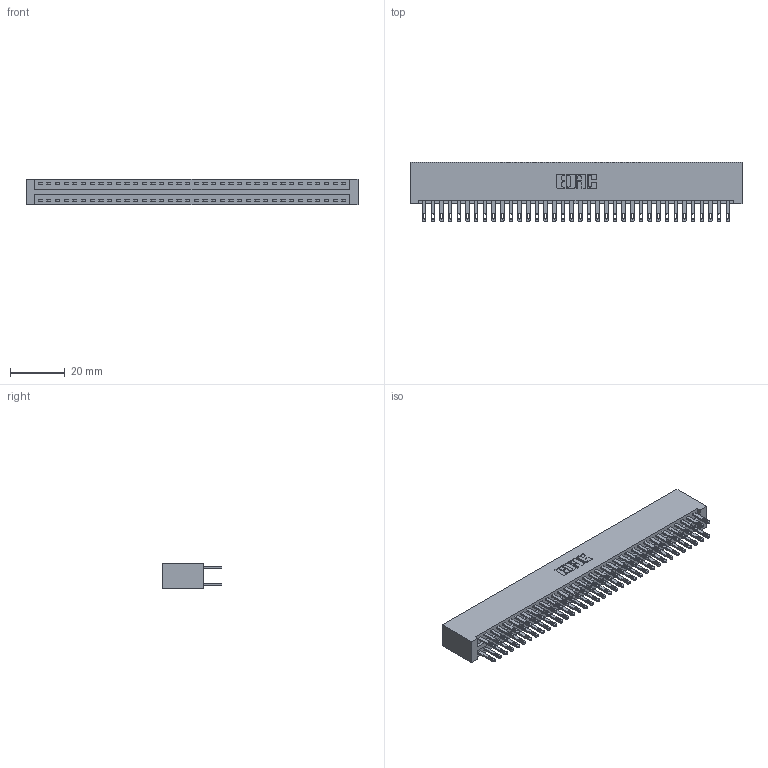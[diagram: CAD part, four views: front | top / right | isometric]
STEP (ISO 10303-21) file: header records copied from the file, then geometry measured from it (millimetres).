
FILE_DESCRIPTION (( 'STEP AP203' ), '1' );
FILE_NAME ('896-072-500-201.STEP', '2021-07-28T01:19:20', ( '' ), ( '' ), 'SwSTEP 2.0', 'SolidWorks 2020', '' );
FILE_SCHEMA (( 'CONFIG_CONTROL_DESIGN' ));
Length unit declared in the file: inch
Products named in the file (3): 345-292-001_345-293-100; 846 Part_No Mounting Lugs; 896-072-500-201
Assembly tree (73 placements, depth 2):
  896-072-500-201
    846 Part_No Mounting Lugs
    345-292-001_345-293-100  x72
Bounding box: 121.54 x 21.84 x 9.4 mm (x, y, z)
Volume: 12598.3 mm3; surface area: 18139.6 mm2
Topology: 73 solids, 73 shells, 3570 faces, 10889 edges, 7258 vertices
Faces by surface type: plane 2160, cylinder 1410
Entity records: 23955 total; most frequent: CARTESIAN_POINT 3952, ORIENTED_EDGE 3886, DIRECTION 3531, EDGE_CURVE 1943, LINE 1671, VECTOR 1671, VERTEX_POINT 1294, AXIS2_PLACEMENT_3D 930
